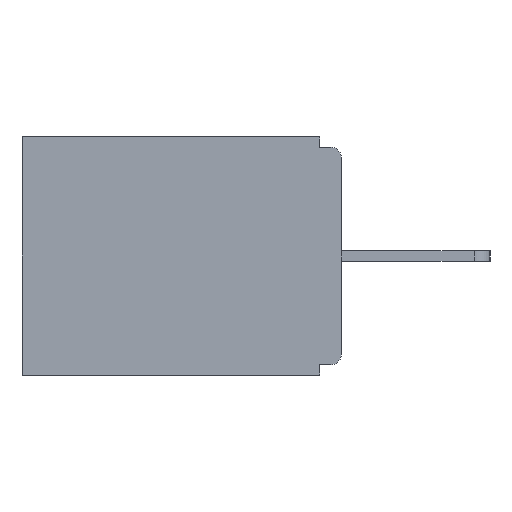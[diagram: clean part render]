
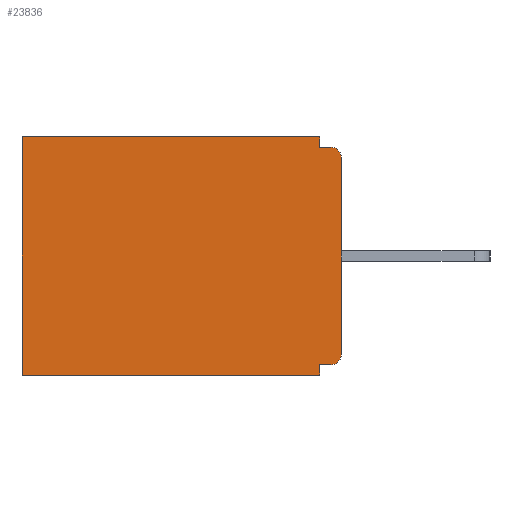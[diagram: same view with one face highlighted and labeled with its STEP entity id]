
A CAD part, left-side view. The second image highlights one B-rep face of the part: STEP entity #23836.
In plain terms, the highlighted planar face has unit normal (-1, 0, 0).
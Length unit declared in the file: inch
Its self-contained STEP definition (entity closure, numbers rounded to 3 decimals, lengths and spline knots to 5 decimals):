
#362 = VECTOR ( 'NONE', #19743, 39.37008 ) ;
#907 = EDGE_CURVE ( 'NONE', #12422, #21207, #5063, .T. ) ;
#1046 = CARTESIAN_POINT ( 'NONE',  ( 0.298, 0.031, -0.343 ) ) ;
#1875 = VECTOR ( 'NONE', #22864, 39.37008 ) ;
#2033 = VERTEX_POINT ( 'NONE', #2923 ) ;
#2174 = ORIENTED_EDGE ( 'NONE', *, *, #16447, .F. ) ;
#2179 = CARTESIAN_POINT ( 'NONE',  ( 0.298, 0., 0. ) ) ;
#2635 = LINE ( 'NONE', #22152, #7504 ) ;
#2923 = CARTESIAN_POINT ( 'NONE',  ( 0.298, 0.031, -0.015 ) ) ;
#3481 = VECTOR ( 'NONE', #15644, 39.37008 ) ;
#3528 = EDGE_LOOP ( 'NONE', ( #17112, #11725, #2174, #5247, #10594, #11873, #10675, #4979, #11294, #16171 ) ) ;
#4441 = EDGE_CURVE ( 'NONE', #16905, #12801, #20065, .T. ) ;
#4452 = LINE ( 'NONE', #20020, #19870 ) ;
#4789 = VECTOR ( 'NONE', #12153, 39.37008 ) ;
#4945 = CARTESIAN_POINT ( 'NONE',  ( 0.298, 0.031, -0.343 ) ) ;
#4979 = ORIENTED_EDGE ( 'NONE', *, *, #8266, .F. ) ;
#5063 = LINE ( 'NONE', #5276, #15161 ) ;
#5242 = CARTESIAN_POINT ( 'NONE',  ( 0.298, 0., -0.343 ) ) ;
#5247 = ORIENTED_EDGE ( 'NONE', *, *, #16811, .T. ) ;
#5276 = CARTESIAN_POINT ( 'NONE',  ( 0.298, 0.46, 0. ) ) ;
#5326 = EDGE_CURVE ( 'NONE', #9088, #14382, #15361, .T. ) ;
#5877 = EDGE_CURVE ( 'NONE', #16905, #14382, #2635, .T. ) ;
#5962 = VERTEX_POINT ( 'NONE', #1046 ) ;
#6362 = DIRECTION ( 'NONE',  ( 1., 0., 0. ) ) ;
#7051 = DIRECTION ( 'NONE',  ( 0., 0., -1. ) ) ;
#7400 = LINE ( 'NONE', #4945, #1875 ) ;
#7504 = VECTOR ( 'NONE', #13721, 39.37008 ) ;
#7586 = CARTESIAN_POINT ( 'NONE',  ( 0.298, 0.015, -0.015 ) ) ;
#8058 = DIRECTION ( 'NONE',  ( -1., 0., 0. ) ) ;
#8266 = EDGE_CURVE ( 'NONE', #9088, #19785, #19558, .T. ) ;
#9010 = VERTEX_POINT ( 'NONE', #24212 ) ;
#9024 = EDGE_CURVE ( 'NONE', #19785, #5962, #16642, .T. ) ;
#9088 = VERTEX_POINT ( 'NONE', #20555 ) ;
#10594 = ORIENTED_EDGE ( 'NONE', *, *, #907, .T. ) ;
#10642 = CARTESIAN_POINT ( 'NONE',  ( 0.298, 0., -0.313 ) ) ;
#10675 = ORIENTED_EDGE ( 'NONE', *, *, #9024, .F. ) ;
#11294 = ORIENTED_EDGE ( 'NONE', *, *, #5326, .T. ) ;
#11725 = ORIENTED_EDGE ( 'NONE', *, *, #12961, .F. ) ;
#11873 = ORIENTED_EDGE ( 'NONE', *, *, #15882, .F. ) ;
#11889 = CARTESIAN_POINT ( 'NONE',  ( 0.298, 0.031, -0.328 ) ) ;
#12153 = DIRECTION ( 'NONE',  ( 0., -1., 0. ) ) ;
#12283 = PLANE ( 'NONE',  #20063 ) ;
#12422 = VERTEX_POINT ( 'NONE', #21915 ) ;
#12801 = VERTEX_POINT ( 'NONE', #7586 ) ;
#12859 = DIRECTION ( 'NONE',  ( -1., 0., 0. ) ) ;
#12891 = CARTESIAN_POINT ( 'NONE',  ( 0.298, 0., -0.03 ) ) ;
#12961 = EDGE_CURVE ( 'NONE', #2033, #12801, #25890, .T. ) ;
#13721 = DIRECTION ( 'NONE',  ( 0., 0., -1. ) ) ;
#14382 = VERTEX_POINT ( 'NONE', #10642 ) ;
#14436 = AXIS2_PLACEMENT_3D ( 'NONE', #23243, #12859, #23002 ) ;
#14707 = CARTESIAN_POINT ( 'NONE',  ( 0.298, 0., -0.328 ) ) ;
#15161 = VECTOR ( 'NONE', #7051, 39.37008 ) ;
#15303 = DIRECTION ( 'NONE',  ( 0., 1., 0. ) ) ;
#15361 = CIRCLE ( 'NONE', #22212, 0.015 ) ;
#15644 = DIRECTION ( 'NONE',  ( 0., 1., 0. ) ) ;
#15882 = EDGE_CURVE ( 'NONE', #5962, #21207, #17127, .T. ) ;
#16171 = ORIENTED_EDGE ( 'NONE', *, *, #5877, .F. ) ;
#16294 = DIRECTION ( 'NONE',  ( 0., 0., -1. ) ) ;
#16406 = CARTESIAN_POINT ( 'NONE',  ( 0.298, 0.46, -0.343 ) ) ;
#16447 = EDGE_CURVE ( 'NONE', #9010, #2033, #7400, .T. ) ;
#16501 = VECTOR ( 'NONE', #15303, 39.37008 ) ;
#16642 = LINE ( 'NONE', #19655, #362 ) ;
#16811 = EDGE_CURVE ( 'NONE', #9010, #12422, #4452, .T. ) ;
#16905 = VERTEX_POINT ( 'NONE', #12891 ) ;
#17021 = FACE_OUTER_BOUND ( 'NONE', #3528, .T. ) ;
#17112 = ORIENTED_EDGE ( 'NONE', *, *, #4441, .T. ) ;
#17127 = LINE ( 'NONE', #5242, #16501 ) ;
#19558 = LINE ( 'NONE', #14707, #3481 ) ;
#19655 = CARTESIAN_POINT ( 'NONE',  ( 0.298, 0.031, -0.343 ) ) ;
#19743 = DIRECTION ( 'NONE',  ( 0., 0., -1. ) ) ;
#19785 = VERTEX_POINT ( 'NONE', #11889 ) ;
#19870 = VECTOR ( 'NONE', #25821, 39.37008 ) ;
#20020 = CARTESIAN_POINT ( 'NONE',  ( 0.298, 0., 0. ) ) ;
#20063 = AXIS2_PLACEMENT_3D ( 'NONE', #2179, #6362, #20345 ) ;
#20065 = CIRCLE ( 'NONE', #14436, 0.015 ) ;
#20345 = DIRECTION ( 'NONE',  ( 0., 0., -1. ) ) ;
#20555 = CARTESIAN_POINT ( 'NONE',  ( 0.298, 0.015, -0.328 ) ) ;
#21207 = VERTEX_POINT ( 'NONE', #16406 ) ;
#21915 = CARTESIAN_POINT ( 'NONE',  ( 0.298, 0.46, 0. ) ) ;
#22152 = CARTESIAN_POINT ( 'NONE',  ( 0.298, 0., 0. ) ) ;
#22212 = AXIS2_PLACEMENT_3D ( 'NONE', #22296, #8058, #16294 ) ;
#22296 = CARTESIAN_POINT ( 'NONE',  ( 0.298, 0.015, -0.313 ) ) ;
#22864 = DIRECTION ( 'NONE',  ( 0., 0., -1. ) ) ;
#23002 = DIRECTION ( 'NONE',  ( 0., 0., -1. ) ) ;
#23243 = CARTESIAN_POINT ( 'NONE',  ( 0.298, 0.015, -0.03 ) ) ;
#23812 = CARTESIAN_POINT ( 'NONE',  ( 0.298, 0., -0.015 ) ) ;
#23836 = ADVANCED_FACE ( 'NONE', ( #17021 ), #12283, .F. ) ;
#24212 = CARTESIAN_POINT ( 'NONE',  ( 0.298, 0.031, 0. ) ) ;
#25821 = DIRECTION ( 'NONE',  ( 0., 1., 0. ) ) ;
#25890 = LINE ( 'NONE', #23812, #4789 ) ;
